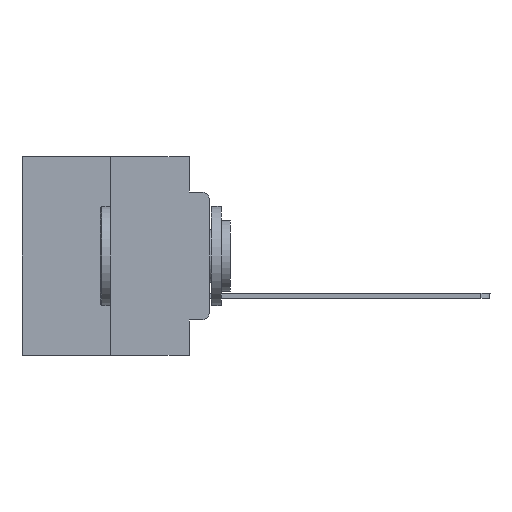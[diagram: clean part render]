
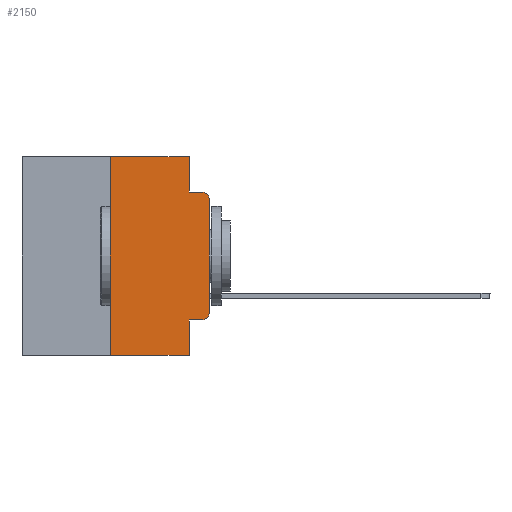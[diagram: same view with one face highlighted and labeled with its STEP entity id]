
A CAD part, left-side view. The second image highlights one B-rep face of the part: STEP entity #2150.
In plain terms, the highlighted planar face has unit normal (-1, 0, 0).
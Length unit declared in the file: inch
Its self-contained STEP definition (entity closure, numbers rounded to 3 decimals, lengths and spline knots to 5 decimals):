
#248 = PLANE ( 'NONE',  #8859 ) ;
#387 = FACE_OUTER_BOUND ( 'NONE', #25568, .T. ) ;
#1312 = CARTESIAN_POINT ( 'NONE',  ( 0., 0.02, -0.1085 ) ) ;
#1721 = ORIENTED_EDGE ( 'NONE', *, *, #19749, .F. ) ;
#1835 = ORIENTED_EDGE ( 'NONE', *, *, #5431, .F. ) ;
#1951 = ORIENTED_EDGE ( 'NONE', *, *, #9862, .F. ) ;
#2150 = ADVANCED_FACE ( 'NONE', ( #387 ), #248, .F. ) ;
#2260 = VERTEX_POINT ( 'NONE', #14858 ) ;
#2337 = DIRECTION ( 'NONE',  ( 1., 0., 0. ) ) ;
#2663 = CARTESIAN_POINT ( 'NONE',  ( 0., 0.051, -0.4115 ) ) ;
#2807 = ORIENTED_EDGE ( 'NONE', *, *, #6377, .T. ) ;
#3461 = EDGE_CURVE ( 'NONE', #17346, #19831, #8457, .T. ) ;
#3691 = EDGE_CURVE ( 'NONE', #10215, #14999, #16876, .T. ) ;
#4135 = VECTOR ( 'NONE', #22622, 39.37008 ) ;
#4327 = LINE ( 'NONE', #6145, #8245 ) ;
#4430 = CARTESIAN_POINT ( 'NONE',  ( 0., 0.473, 0. ) ) ;
#5431 = EDGE_CURVE ( 'NONE', #10232, #14999, #8070, .T. ) ;
#5852 = VECTOR ( 'NONE', #17687, 39.37008 ) ;
#6145 = CARTESIAN_POINT ( 'NONE',  ( 0., 0.051, 0. ) ) ;
#6176 = DIRECTION ( 'NONE',  ( 0., 0., -1. ) ) ;
#6377 = EDGE_CURVE ( 'NONE', #18660, #24674, #25686, .T. ) ;
#6697 = LINE ( 'NONE', #15180, #25685 ) ;
#6722 = CARTESIAN_POINT ( 'NONE',  ( 0., 0.02, -0.3915 ) ) ;
#7309 = ORIENTED_EDGE ( 'NONE', *, *, #15491, .F. ) ;
#7495 = CARTESIAN_POINT ( 'NONE',  ( 0., 0., -0.1085 ) ) ;
#8070 = LINE ( 'NONE', #15036, #26208 ) ;
#8245 = VECTOR ( 'NONE', #25612, 39.37008 ) ;
#8457 = LINE ( 'NONE', #4430, #17764 ) ;
#8859 = AXIS2_PLACEMENT_3D ( 'NONE', #15138, #2337, #17226 ) ;
#9794 = DIRECTION ( 'NONE',  ( -1., 0., 0. ) ) ;
#9862 = EDGE_CURVE ( 'NONE', #16774, #17346, #15154, .T. ) ;
#10215 = VERTEX_POINT ( 'NONE', #7495 ) ;
#10232 = VERTEX_POINT ( 'NONE', #20315 ) ;
#10323 = CARTESIAN_POINT ( 'NONE',  ( 0., 0.25, -0.5 ) ) ;
#10582 = EDGE_CURVE ( 'NONE', #16774, #2260, #24432, .T. ) ;
#12377 = CARTESIAN_POINT ( 'NONE',  ( 0., 0., -0.3915 ) ) ;
#13097 = DIRECTION ( 'NONE',  ( 0., 0., -1. ) ) ;
#14330 = ORIENTED_EDGE ( 'NONE', *, *, #3691, .T. ) ;
#14858 = CARTESIAN_POINT ( 'NONE',  ( 0., 0.051, -0.5 ) ) ;
#14999 = VERTEX_POINT ( 'NONE', #18977 ) ;
#15036 = CARTESIAN_POINT ( 'NONE',  ( 0., 0.051, -0.0885 ) ) ;
#15138 = CARTESIAN_POINT ( 'NONE',  ( 0., 0.473, 0. ) ) ;
#15154 = LINE ( 'NONE', #23637, #18761 ) ;
#15180 = CARTESIAN_POINT ( 'NONE',  ( 0., 0.051, 0. ) ) ;
#15208 = DIRECTION ( 'NONE',  ( -1., 0., 0. ) ) ;
#15297 = CARTESIAN_POINT ( 'NONE',  ( 0., 0.25, 0. ) ) ;
#15491 = EDGE_CURVE ( 'NONE', #19831, #10232, #4327, .T. ) ;
#16410 = DIRECTION ( 'NONE',  ( 0., 0., 1. ) ) ;
#16734 = ORIENTED_EDGE ( 'NONE', *, *, #3461, .F. ) ;
#16774 = VERTEX_POINT ( 'NONE', #10323 ) ;
#16832 = VERTEX_POINT ( 'NONE', #2663 ) ;
#16859 = CARTESIAN_POINT ( 'NONE',  ( 0., 0.02, -0.4115 ) ) ;
#16876 = CIRCLE ( 'NONE', #18213, 0.02 ) ;
#17226 = DIRECTION ( 'NONE',  ( 0., 0., -1. ) ) ;
#17346 = VERTEX_POINT ( 'NONE', #15297 ) ;
#17687 = DIRECTION ( 'NONE',  ( 0., -1., 0. ) ) ;
#17764 = VECTOR ( 'NONE', #19055, 39.37008 ) ;
#18213 = AXIS2_PLACEMENT_3D ( 'NONE', #1312, #9794, #26754 ) ;
#18660 = VERTEX_POINT ( 'NONE', #16859 ) ;
#18761 = VECTOR ( 'NONE', #21428, 39.37008 ) ;
#18973 = ORIENTED_EDGE ( 'NONE', *, *, #27479, .T. ) ;
#18977 = CARTESIAN_POINT ( 'NONE',  ( 0., 0.02, -0.0885 ) ) ;
#19055 = DIRECTION ( 'NONE',  ( 0., -1., 0. ) ) ;
#19079 = DIRECTION ( 'NONE',  ( 0., -1., 0. ) ) ;
#19749 = EDGE_CURVE ( 'NONE', #16832, #2260, #6697, .T. ) ;
#19831 = VERTEX_POINT ( 'NONE', #25881 ) ;
#20187 = LINE ( 'NONE', #22800, #22479 ) ;
#20315 = CARTESIAN_POINT ( 'NONE',  ( 0., 0.051, -0.0885 ) ) ;
#21428 = DIRECTION ( 'NONE',  ( 0., 0., 1. ) ) ;
#21574 = ORIENTED_EDGE ( 'NONE', *, *, #24522, .T. ) ;
#22004 = CARTESIAN_POINT ( 'NONE',  ( 0., 0.051, -0.4115 ) ) ;
#22479 = VECTOR ( 'NONE', #16410, 39.37008 ) ;
#22622 = DIRECTION ( 'NONE',  ( 0., -1., 0. ) ) ;
#22645 = LINE ( 'NONE', #22004, #5852 ) ;
#22800 = CARTESIAN_POINT ( 'NONE',  ( 0., 0., 0. ) ) ;
#23637 = CARTESIAN_POINT ( 'NONE',  ( 0., 0.25, 0. ) ) ;
#24354 = AXIS2_PLACEMENT_3D ( 'NONE', #6722, #15208, #6176 ) ;
#24432 = LINE ( 'NONE', #26652, #4135 ) ;
#24522 = EDGE_CURVE ( 'NONE', #24674, #10215, #20187, .T. ) ;
#24674 = VERTEX_POINT ( 'NONE', #12377 ) ;
#25568 = EDGE_LOOP ( 'NONE', ( #21574, #14330, #1835, #7309, #16734, #1951, #25678, #1721, #18973, #2807 ) ) ;
#25612 = DIRECTION ( 'NONE',  ( 0., 0., -1. ) ) ;
#25678 = ORIENTED_EDGE ( 'NONE', *, *, #10582, .T. ) ;
#25685 = VECTOR ( 'NONE', #13097, 39.37008 ) ;
#25686 = CIRCLE ( 'NONE', #24354, 0.02 ) ;
#25881 = CARTESIAN_POINT ( 'NONE',  ( 0., 0.051, 0. ) ) ;
#26208 = VECTOR ( 'NONE', #19079, 39.37008 ) ;
#26652 = CARTESIAN_POINT ( 'NONE',  ( 0., 0.473, -0.5 ) ) ;
#26754 = DIRECTION ( 'NONE',  ( 0., 0., -1. ) ) ;
#27479 = EDGE_CURVE ( 'NONE', #16832, #18660, #22645, .T. ) ;
